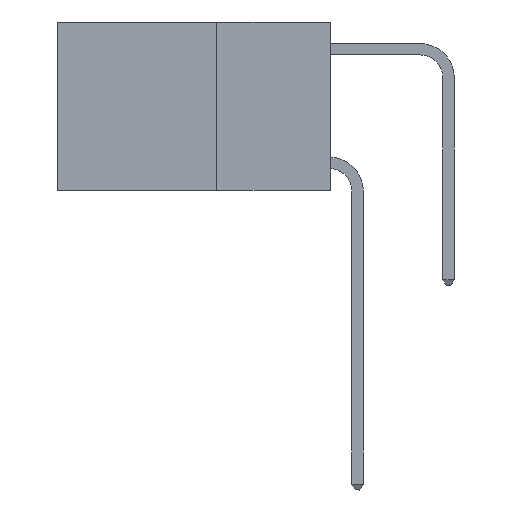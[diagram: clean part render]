
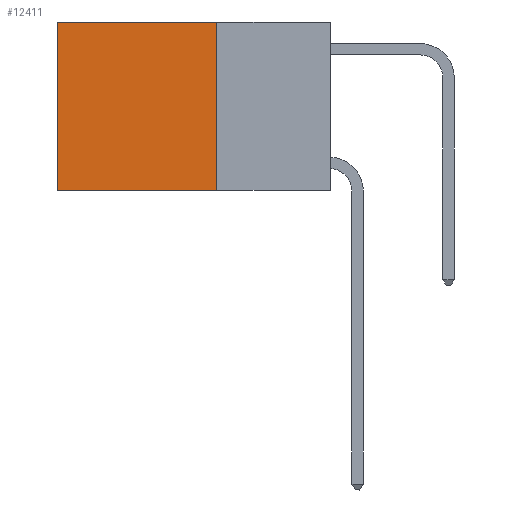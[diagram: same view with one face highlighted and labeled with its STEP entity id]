
A CAD part, left-side view. The second image highlights one B-rep face of the part: STEP entity #12411.
In plain terms, the highlighted planar face has unit normal (-1, 0, 0).
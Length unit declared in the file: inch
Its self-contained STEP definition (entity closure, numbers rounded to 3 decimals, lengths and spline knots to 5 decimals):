
#1325 = DIRECTION ( 'NONE',  ( 0., 0., -1. ) ) ;
#3412 = CARTESIAN_POINT ( 'NONE',  ( 0.2625, 0.25, 0. ) ) ;
#3668 = VERTEX_POINT ( 'NONE', #26567 ) ;
#3949 = EDGE_CURVE ( 'NONE', #7505, #3668, #14761, .T. ) ;
#6371 = LINE ( 'NONE', #15037, #23617 ) ;
#6386 = DIRECTION ( 'NONE',  ( 0., 0., -1. ) ) ;
#6847 = EDGE_CURVE ( 'NONE', #3668, #8143, #6371, .T. ) ;
#7505 = VERTEX_POINT ( 'NONE', #19221 ) ;
#7964 = CARTESIAN_POINT ( 'NONE',  ( 0.2625, 0.25, -0.37 ) ) ;
#8143 = VERTEX_POINT ( 'NONE', #24176 ) ;
#9664 = AXIS2_PLACEMENT_3D ( 'NONE', #21230, #10603, #6386 ) ;
#10603 = DIRECTION ( 'NONE',  ( 1., 0., 0. ) ) ;
#10987 = ORIENTED_EDGE ( 'NONE', *, *, #21679, .F. ) ;
#12079 = CARTESIAN_POINT ( 'NONE',  ( 0.2625, 0.25, -0.37 ) ) ;
#12411 = ADVANCED_FACE ( 'NONE', ( #25596 ), #20821, .F. ) ;
#12661 = CARTESIAN_POINT ( 'NONE',  ( 0.2625, 0.25, 0. ) ) ;
#14761 = LINE ( 'NONE', #12661, #24491 ) ;
#15037 = CARTESIAN_POINT ( 'NONE',  ( 0.2625, 0.6, 0. ) ) ;
#15837 = LINE ( 'NONE', #12079, #23532 ) ;
#16122 = VECTOR ( 'NONE', #1325, 39.37008 ) ;
#16364 = VERTEX_POINT ( 'NONE', #7964 ) ;
#16621 = ORIENTED_EDGE ( 'NONE', *, *, #3949, .T. ) ;
#17632 = ORIENTED_EDGE ( 'NONE', *, *, #21302, .F. ) ;
#19221 = CARTESIAN_POINT ( 'NONE',  ( 0.2625, 0.25, 0. ) ) ;
#20821 = PLANE ( 'NONE',  #9664 ) ;
#21193 = DIRECTION ( 'NONE',  ( 0., 1., 0. ) ) ;
#21230 = CARTESIAN_POINT ( 'NONE',  ( 0.2625, 0.25, 0. ) ) ;
#21302 = EDGE_CURVE ( 'NONE', #7505, #16364, #24577, .T. ) ;
#21624 = DIRECTION ( 'NONE',  ( 0., 0., -1. ) ) ;
#21679 = EDGE_CURVE ( 'NONE', #16364, #8143, #15837, .T. ) ;
#22145 = DIRECTION ( 'NONE',  ( 0., 1., 0. ) ) ;
#23532 = VECTOR ( 'NONE', #22145, 39.37008 ) ;
#23617 = VECTOR ( 'NONE', #21624, 39.37008 ) ;
#24176 = CARTESIAN_POINT ( 'NONE',  ( 0.2625, 0.6, -0.37 ) ) ;
#24369 = EDGE_LOOP ( 'NONE', ( #27203, #10987, #17632, #16621 ) ) ;
#24491 = VECTOR ( 'NONE', #21193, 39.37008 ) ;
#24577 = LINE ( 'NONE', #3412, #16122 ) ;
#25596 = FACE_OUTER_BOUND ( 'NONE', #24369, .T. ) ;
#26567 = CARTESIAN_POINT ( 'NONE',  ( 0.2625, 0.6, 0. ) ) ;
#27203 = ORIENTED_EDGE ( 'NONE', *, *, #6847, .T. ) ;
